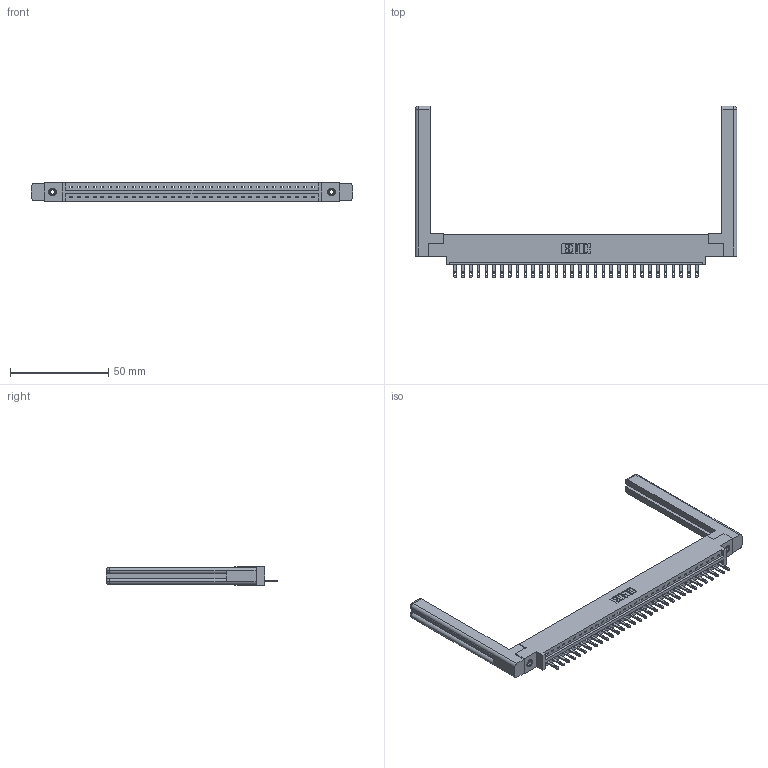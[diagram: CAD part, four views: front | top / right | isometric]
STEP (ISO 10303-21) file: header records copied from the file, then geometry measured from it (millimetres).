
FILE_DESCRIPTION (( 'STEP AP203' ), '1' );
FILE_NAME ('337-032-500-658.STEP', '2019-10-01T02:19:34', ( '' ), ( '' ), 'SwSTEP 2.0', 'SolidWorks 2016', '' );
FILE_SCHEMA (( 'CONFIG_CONTROL_DESIGN' ));
Length unit declared in the file: inch
Products named in the file (5): 345-292-001_345-293-100; 337-032-500-658; 307-220-058; 337 Part_0.170 Offset - 0.156 Dia-TI; 345-250-001_345-250-001-102
Assembly tree (37 placements, depth 2):
  337-032-500-658
    337 Part_0.170 Offset - 0.156 Dia-TI
    345-292-001_345-293-100  x32
    345-250-001_345-250-001-102  x2
    307-220-058  x2
Bounding box: 163.42 x 87.25 x 9.4 mm (x, y, z)
Volume: 23924.5 mm3; surface area: 22650 mm2
Topology: 37 solids, 37 shells, 2116 faces, 6437 edges, 4278 vertices
Faces by surface type: plane 1438, cylinder 654, cone 12, torus 12
Entity records: 27776 total; most frequent: CARTESIAN_POINT 4837, ORIENTED_EDGE 4744, DIRECTION 4112, EDGE_CURVE 2372, LINE 2192, VECTOR 2192, VERTEX_POINT 1574, AXIS2_PLACEMENT_3D 960
